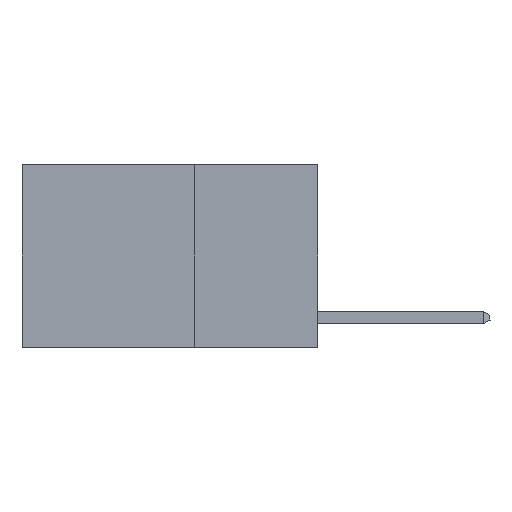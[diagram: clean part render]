
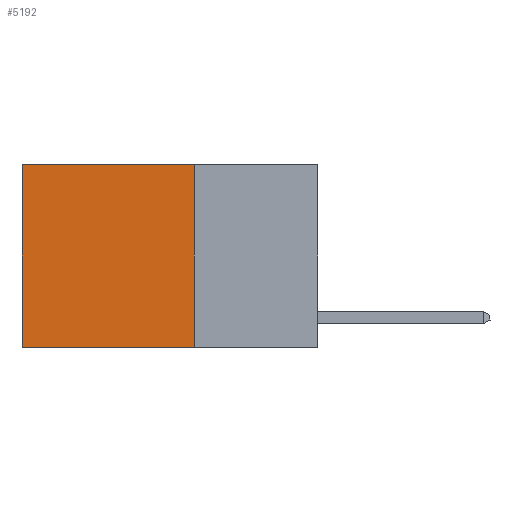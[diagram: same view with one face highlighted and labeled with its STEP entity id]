
A CAD part, left-side view. The second image highlights one B-rep face of the part: STEP entity #5192.
In plain terms, the highlighted planar face has unit normal (-1, 0, 0).
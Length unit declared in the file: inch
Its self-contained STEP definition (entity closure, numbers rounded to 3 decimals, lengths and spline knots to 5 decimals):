
#110 = DIRECTION ( 'NONE',  ( 0., 1., 0. ) ) ;
#125 = ORIENTED_EDGE ( 'NONE', *, *, #8935, .F. ) ;
#424 = EDGE_CURVE ( 'NONE', #12242, #15910, #3342, .T. ) ;
#791 = CARTESIAN_POINT ( 'NONE',  ( 0.2625, 0.25, 0. ) ) ;
#815 = DIRECTION ( 'NONE',  ( 0., 0., -1. ) ) ;
#1248 = FACE_OUTER_BOUND ( 'NONE', #2186, .T. ) ;
#1767 = ORIENTED_EDGE ( 'NONE', *, *, #424, .F. ) ;
#1856 = DIRECTION ( 'NONE',  ( 0., 1., 0. ) ) ;
#1872 = ORIENTED_EDGE ( 'NONE', *, *, #10114, .T. ) ;
#2186 = EDGE_LOOP ( 'NONE', ( #15948, #1767, #125, #1872 ) ) ;
#2206 = LINE ( 'NONE', #11770, #17222 ) ;
#2764 = CARTESIAN_POINT ( 'NONE',  ( 0.2625, 0.25, -0.37 ) ) ;
#3342 = LINE ( 'NONE', #12810, #17443 ) ;
#3440 = PLANE ( 'NONE',  #10719 ) ;
#4255 = VECTOR ( 'NONE', #12141, 39.37008 ) ;
#5192 = ADVANCED_FACE ( 'NONE', ( #1248 ), #3440, .F. ) ;
#5695 = VERTEX_POINT ( 'NONE', #6129 ) ;
#6129 = CARTESIAN_POINT ( 'NONE',  ( 0.2625, 0.6, 0. ) ) ;
#6327 = DIRECTION ( 'NONE',  ( 0., 0., -1. ) ) ;
#6451 = EDGE_CURVE ( 'NONE', #5695, #15910, #7252, .T. ) ;
#7252 = LINE ( 'NONE', #10639, #9638 ) ;
#8935 = EDGE_CURVE ( 'NONE', #18204, #12242, #12675, .T. ) ;
#9638 = VECTOR ( 'NONE', #815, 39.37008 ) ;
#10114 = EDGE_CURVE ( 'NONE', #18204, #5695, #2206, .T. ) ;
#10639 = CARTESIAN_POINT ( 'NONE',  ( 0.2625, 0.6, 0. ) ) ;
#10719 = AXIS2_PLACEMENT_3D ( 'NONE', #13325, #14743, #6327 ) ;
#11770 = CARTESIAN_POINT ( 'NONE',  ( 0.2625, 0.25, 0. ) ) ;
#12141 = DIRECTION ( 'NONE',  ( 0., 0., -1. ) ) ;
#12242 = VERTEX_POINT ( 'NONE', #2764 ) ;
#12675 = LINE ( 'NONE', #791, #4255 ) ;
#12810 = CARTESIAN_POINT ( 'NONE',  ( 0.2625, 0.25, -0.37 ) ) ;
#13325 = CARTESIAN_POINT ( 'NONE',  ( 0.2625, 0.25, 0. ) ) ;
#14743 = DIRECTION ( 'NONE',  ( 1., 0., 0. ) ) ;
#14860 = CARTESIAN_POINT ( 'NONE',  ( 0.2625, 0.25, 0. ) ) ;
#15558 = CARTESIAN_POINT ( 'NONE',  ( 0.2625, 0.6, -0.37 ) ) ;
#15910 = VERTEX_POINT ( 'NONE', #15558 ) ;
#15948 = ORIENTED_EDGE ( 'NONE', *, *, #6451, .T. ) ;
#17222 = VECTOR ( 'NONE', #1856, 39.37008 ) ;
#17443 = VECTOR ( 'NONE', #110, 39.37008 ) ;
#18204 = VERTEX_POINT ( 'NONE', #14860 ) ;
